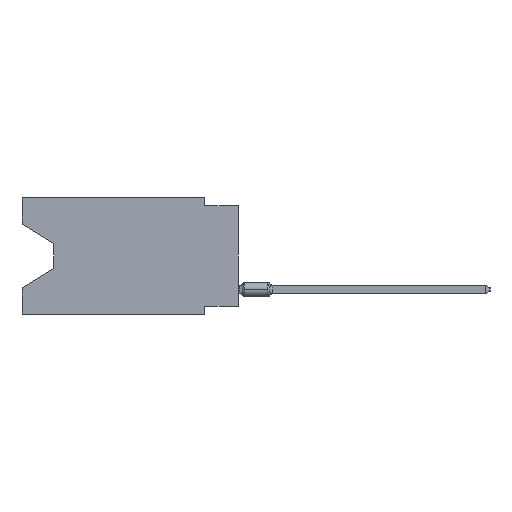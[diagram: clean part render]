
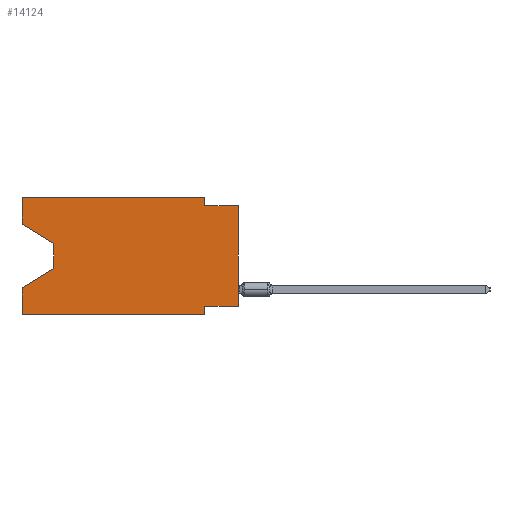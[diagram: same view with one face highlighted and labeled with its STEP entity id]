
A CAD part, left-side view. The second image highlights one B-rep face of the part: STEP entity #14124.
In plain terms, the highlighted planar face has unit normal (-1, 0, 0).
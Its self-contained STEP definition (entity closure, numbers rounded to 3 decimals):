
#184 = CARTESIAN_POINT ( 'NONE',  ( 0., 16.383, -8.89 ) ) ;
#433 = CARTESIAN_POINT ( 'NONE',  ( 0., 16.383, -6.852 ) ) ;
#719 = VERTEX_POINT ( 'NONE', #61073 ) ;
#1808 = CARTESIAN_POINT ( 'NONE',  ( 0., 0., -8.255 ) ) ;
#3768 = CARTESIAN_POINT ( 'NONE',  ( 0., 0., -0.635 ) ) ;
#4027 = DIRECTION ( 'NONE',  ( 0., -1., 0. ) ) ;
#4509 = EDGE_CURVE ( 'NONE', #719, #17256, #57519, .T. ) ;
#4810 = VERTEX_POINT ( 'NONE', #3768 ) ;
#4975 = VECTOR ( 'NONE', #4027, 1000. ) ;
#5119 = ORIENTED_EDGE ( 'NONE', *, *, #55883, .T. ) ;
#5502 = EDGE_CURVE ( 'NONE', #17256, #54846, #6576, .T. ) ;
#5534 = CARTESIAN_POINT ( 'NONE',  ( 0., 13.97, -3.505 ) ) ;
#5576 = ORIENTED_EDGE ( 'NONE', *, *, #27056, .F. ) ;
#5967 = DIRECTION ( 'NONE',  ( 0., 0., -1. ) ) ;
#6161 = ORIENTED_EDGE ( 'NONE', *, *, #49233, .F. ) ;
#6372 = AXIS2_PLACEMENT_3D ( 'NONE', #43943, #15247, #34361 ) ;
#6576 = LINE ( 'NONE', #14866, #60118 ) ;
#9440 = CARTESIAN_POINT ( 'NONE',  ( 0., 16.383, -2.038 ) ) ;
#10803 = ORIENTED_EDGE ( 'NONE', *, *, #33908, .T. ) ;
#10903 = CARTESIAN_POINT ( 'NONE',  ( 0., 16.383, 0. ) ) ;
#12094 = CARTESIAN_POINT ( 'NONE',  ( 0., 13.97, -5.385 ) ) ;
#12573 = VERTEX_POINT ( 'NONE', #433 ) ;
#14003 = ORIENTED_EDGE ( 'NONE', *, *, #17867, .T. ) ;
#14124 = ADVANCED_FACE ( 'NONE', ( #19721 ), #29269, .F. ) ;
#14494 = VECTOR ( 'NONE', #5967, 1000. ) ;
#14866 = CARTESIAN_POINT ( 'NONE',  ( 0., 13.97, -3.505 ) ) ;
#15247 = DIRECTION ( 'NONE',  ( 1., 0., 0. ) ) ;
#17256 = VERTEX_POINT ( 'NONE', #5534 ) ;
#17867 = EDGE_CURVE ( 'NONE', #54846, #12573, #26100, .T. ) ;
#18085 = VECTOR ( 'NONE', #35777, 1000. ) ;
#18572 = ORIENTED_EDGE ( 'NONE', *, *, #29152, .F. ) ;
#19309 = EDGE_LOOP ( 'NONE', ( #60860, #42652, #14003, #18572, #5119, #39533, #45583, #10803, #33429, #5576, #6161, #36417 ) ) ;
#19396 = VERTEX_POINT ( 'NONE', #33409 ) ;
#19480 = VECTOR ( 'NONE', #25425, 1000. ) ;
#19721 = FACE_OUTER_BOUND ( 'NONE', #19309, .T. ) ;
#20415 = DIRECTION ( 'NONE',  ( 0., 0.855, -0.519 ) ) ;
#20840 = VECTOR ( 'NONE', #49865, 1000. ) ;
#21090 = CARTESIAN_POINT ( 'NONE',  ( 0., 2.54, -8.89 ) ) ;
#22319 = EDGE_CURVE ( 'NONE', #719, #35611, #22922, .T. ) ;
#22922 = LINE ( 'NONE', #37245, #32487 ) ;
#25344 = DIRECTION ( 'NONE',  ( 0., -1., 0. ) ) ;
#25425 = DIRECTION ( 'NONE',  ( 0., -1., 0. ) ) ;
#25657 = CARTESIAN_POINT ( 'NONE',  ( 0., 0., -8.255 ) ) ;
#25684 = DIRECTION ( 'NONE',  ( 0., 0., -1. ) ) ;
#25782 = CARTESIAN_POINT ( 'NONE',  ( 0., 2.54, -8.89 ) ) ;
#26100 = LINE ( 'NONE', #12094, #53580 ) ;
#27056 = EDGE_CURVE ( 'NONE', #41084, #28593, #53131, .T. ) ;
#27168 = LINE ( 'NONE', #36089, #18085 ) ;
#27219 = VERTEX_POINT ( 'NONE', #1808 ) ;
#28482 = VERTEX_POINT ( 'NONE', #25782 ) ;
#28593 = VERTEX_POINT ( 'NONE', #56047 ) ;
#29152 = EDGE_CURVE ( 'NONE', #19396, #12573, #35104, .T. ) ;
#29269 = PLANE ( 'NONE',  #6372 ) ;
#30114 = LINE ( 'NONE', #54025, #55063 ) ;
#30817 = VERTEX_POINT ( 'NONE', #32469 ) ;
#31240 = CARTESIAN_POINT ( 'NONE',  ( 0., 13.97, -5.385 ) ) ;
#31520 = EDGE_CURVE ( 'NONE', #27219, #30817, #59745, .T. ) ;
#32469 = CARTESIAN_POINT ( 'NONE',  ( 0., 2.54, -8.255 ) ) ;
#32487 = VECTOR ( 'NONE', #56065, 1000. ) ;
#33409 = CARTESIAN_POINT ( 'NONE',  ( 0., 16.383, -8.89 ) ) ;
#33429 = ORIENTED_EDGE ( 'NONE', *, *, #58896, .F. ) ;
#33908 = EDGE_CURVE ( 'NONE', #27219, #4810, #27168, .T. ) ;
#34361 = DIRECTION ( 'NONE',  ( 0., 0., -1. ) ) ;
#35104 = LINE ( 'NONE', #10903, #51267 ) ;
#35611 = VERTEX_POINT ( 'NONE', #37917 ) ;
#35777 = DIRECTION ( 'NONE',  ( 0., 0., 1. ) ) ;
#36089 = CARTESIAN_POINT ( 'NONE',  ( 0., 0., 0. ) ) ;
#36417 = ORIENTED_EDGE ( 'NONE', *, *, #22319, .F. ) ;
#37245 = CARTESIAN_POINT ( 'NONE',  ( 0., 16.383, 0. ) ) ;
#37693 = VECTOR ( 'NONE', #45007, 1000. ) ;
#37917 = CARTESIAN_POINT ( 'NONE',  ( 0., 16.383, 0. ) ) ;
#39533 = ORIENTED_EDGE ( 'NONE', *, *, #57731, .F. ) ;
#41084 = VERTEX_POINT ( 'NONE', #43321 ) ;
#41587 = LINE ( 'NONE', #49322, #19480 ) ;
#42652 = ORIENTED_EDGE ( 'NONE', *, *, #5502, .T. ) ;
#43321 = CARTESIAN_POINT ( 'NONE',  ( 0., 2.54, 0. ) ) ;
#43943 = CARTESIAN_POINT ( 'NONE',  ( 0., 16.383, 0. ) ) ;
#44679 = DIRECTION ( 'NONE',  ( 0., 0., 1. ) ) ;
#44688 = LINE ( 'NONE', #21090, #37693 ) ;
#45007 = DIRECTION ( 'NONE',  ( 0., 0., -1. ) ) ;
#45583 = ORIENTED_EDGE ( 'NONE', *, *, #31520, .F. ) ;
#49233 = EDGE_CURVE ( 'NONE', #35611, #41084, #41587, .T. ) ;
#49322 = CARTESIAN_POINT ( 'NONE',  ( 0., 16.383, 0. ) ) ;
#49865 = DIRECTION ( 'NONE',  ( 0., 1., 0. ) ) ;
#51267 = VECTOR ( 'NONE', #44679, 1000. ) ;
#53131 = LINE ( 'NONE', #63001, #14494 ) ;
#53580 = VECTOR ( 'NONE', #20415, 1000. ) ;
#54025 = CARTESIAN_POINT ( 'NONE',  ( 0., 0., -0.635 ) ) ;
#54846 = VERTEX_POINT ( 'NONE', #31240 ) ;
#55063 = VECTOR ( 'NONE', #25344, 1000. ) ;
#55883 = EDGE_CURVE ( 'NONE', #19396, #28482, #57136, .T. ) ;
#56047 = CARTESIAN_POINT ( 'NONE',  ( 0., 2.54, -0.635 ) ) ;
#56065 = DIRECTION ( 'NONE',  ( 0., 0., 1. ) ) ;
#57136 = LINE ( 'NONE', #184, #4975 ) ;
#57519 = LINE ( 'NONE', #9440, #57977 ) ;
#57731 = EDGE_CURVE ( 'NONE', #30817, #28482, #44688, .T. ) ;
#57977 = VECTOR ( 'NONE', #62932, 1000. ) ;
#58896 = EDGE_CURVE ( 'NONE', #28593, #4810, #30114, .T. ) ;
#59745 = LINE ( 'NONE', #25657, #20840 ) ;
#60118 = VECTOR ( 'NONE', #25684, 1000. ) ;
#60860 = ORIENTED_EDGE ( 'NONE', *, *, #4509, .T. ) ;
#61073 = CARTESIAN_POINT ( 'NONE',  ( 0., 16.383, -2.038 ) ) ;
#62932 = DIRECTION ( 'NONE',  ( 0., -0.855, -0.519 ) ) ;
#63001 = CARTESIAN_POINT ( 'NONE',  ( 0., 2.54, 0. ) ) ;
